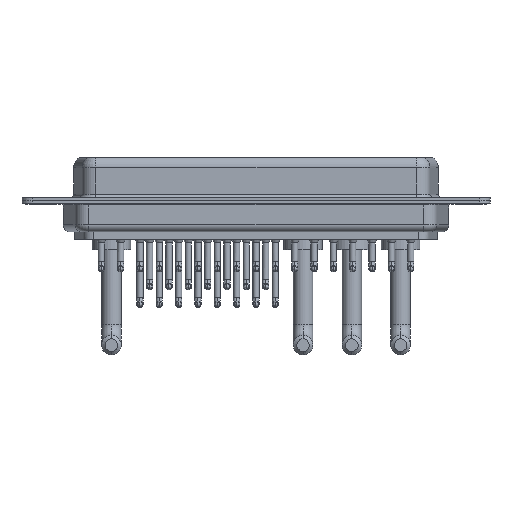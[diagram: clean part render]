
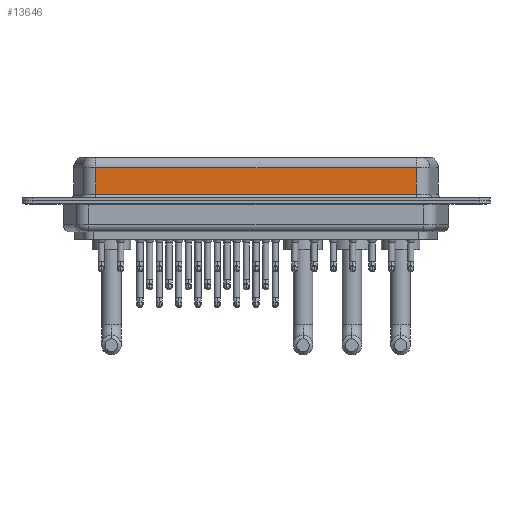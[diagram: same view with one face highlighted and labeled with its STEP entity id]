
A CAD part, front view. The second image highlights one B-rep face of the part: STEP entity #13646.
In plain terms, the highlighted planar face has unit normal (0, -1, 0).
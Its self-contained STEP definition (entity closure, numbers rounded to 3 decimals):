
#454 = DIRECTION ( 'NONE',  ( 0., 1., 0. ) ) ;
#553 = VERTEX_POINT ( 'NONE', #18793 ) ;
#1190 = EDGE_LOOP ( 'NONE', ( #25179, #1904, #12908, #26321 ) ) ;
#1904 = ORIENTED_EDGE ( 'NONE', *, *, #12530, .T. ) ;
#2529 = LINE ( 'NONE', #15674, #12992 ) ;
#4955 = AXIS2_PLACEMENT_3D ( 'NONE', #11077, #454, #10942 ) ;
#5294 = CARTESIAN_POINT ( 'NONE',  ( 7.59, -5.375, 4.65 ) ) ;
#6119 = DIRECTION ( 'NONE',  ( 1., 0., 0. ) ) ;
#9206 = EDGE_CURVE ( 'NONE', #19975, #18744, #26109, .T. ) ;
#9274 = DIRECTION ( 'NONE',  ( 0., 0., -1. ) ) ;
#9394 = CARTESIAN_POINT ( 'NONE',  ( 7.59, -5.375, 6.4 ) ) ;
#10595 = VECTOR ( 'NONE', #9274, 1000. ) ;
#10758 = VECTOR ( 'NONE', #6119, 1000. ) ;
#10942 = DIRECTION ( 'NONE',  ( 0., 0., 1. ) ) ;
#11077 = CARTESIAN_POINT ( 'NONE',  ( 53.41, -5.375, 6.4 ) ) ;
#12530 = EDGE_CURVE ( 'NONE', #19975, #26498, #2529, .T. ) ;
#12908 = ORIENTED_EDGE ( 'NONE', *, *, #13864, .T. ) ;
#12992 = VECTOR ( 'NONE', #25955, 1000. ) ;
#13646 = ADVANCED_FACE ( 'NONE', ( #21222 ), #25809, .F. ) ;
#13864 = EDGE_CURVE ( 'NONE', #26498, #553, #24016, .T. ) ;
#15674 = CARTESIAN_POINT ( 'NONE',  ( 53.41, -5.375, 4.65 ) ) ;
#15679 = DIRECTION ( 'NONE',  ( 0., 0., -1. ) ) ;
#17001 = VECTOR ( 'NONE', #15679, 1000. ) ;
#17585 = CARTESIAN_POINT ( 'NONE',  ( 53.41, -5.375, 0.9 ) ) ;
#18565 = CARTESIAN_POINT ( 'NONE',  ( 53.41, -5.375, 4.65 ) ) ;
#18744 = VERTEX_POINT ( 'NONE', #17585 ) ;
#18793 = CARTESIAN_POINT ( 'NONE',  ( 7.59, -5.375, 0.9 ) ) ;
#19975 = VERTEX_POINT ( 'NONE', #18565 ) ;
#21222 = FACE_OUTER_BOUND ( 'NONE', #1190, .T. ) ;
#21808 = CARTESIAN_POINT ( 'NONE',  ( 53.41, -5.375, 6.4 ) ) ;
#24016 = LINE ( 'NONE', #9394, #17001 ) ;
#25070 = LINE ( 'NONE', #25195, #10758 ) ;
#25179 = ORIENTED_EDGE ( 'NONE', *, *, #9206, .F. ) ;
#25195 = CARTESIAN_POINT ( 'NONE',  ( 53.41, -5.375, 0.9 ) ) ;
#25809 = PLANE ( 'NONE',  #4955 ) ;
#25955 = DIRECTION ( 'NONE',  ( -1., 0., 0. ) ) ;
#26109 = LINE ( 'NONE', #21808, #10595 ) ;
#26321 = ORIENTED_EDGE ( 'NONE', *, *, #26688, .T. ) ;
#26498 = VERTEX_POINT ( 'NONE', #5294 ) ;
#26688 = EDGE_CURVE ( 'NONE', #553, #18744, #25070, .T. ) ;
